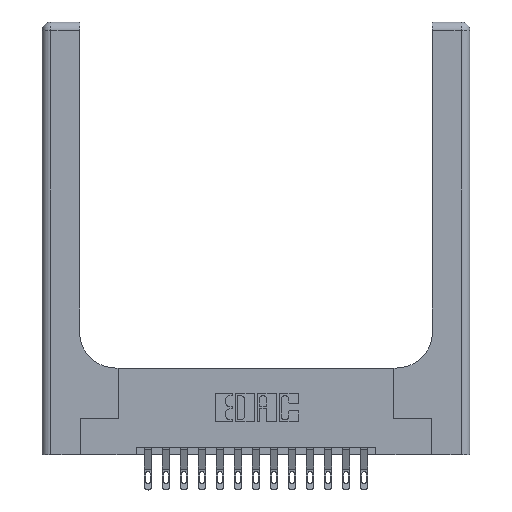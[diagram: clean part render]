
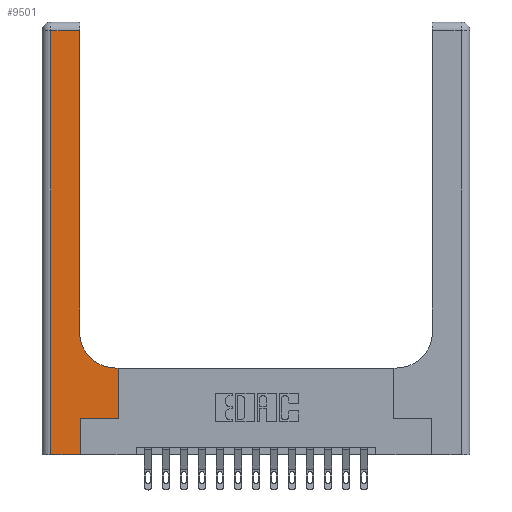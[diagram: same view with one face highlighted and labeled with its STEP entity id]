
A CAD part, top view. The second image highlights one B-rep face of the part: STEP entity #9501.
In plain terms, the highlighted planar face has unit normal (0, 0, 1).
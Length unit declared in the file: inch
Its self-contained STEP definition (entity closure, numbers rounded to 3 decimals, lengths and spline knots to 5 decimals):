
#253 = VECTOR ( 'NONE', #8707, 39.37008 ) ;
#255 = VERTEX_POINT ( 'NONE', #15334 ) ;
#496 = VERTEX_POINT ( 'NONE', #16063 ) ;
#743 = EDGE_CURVE ( 'NONE', #5864, #2166, #17079, .T. ) ;
#799 = CIRCLE ( 'NONE', #3580, 0.25 ) ;
#1097 = ORIENTED_EDGE ( 'NONE', *, *, #6140, .T. ) ;
#2155 = EDGE_CURVE ( 'NONE', #9867, #15164, #10991, .T. ) ;
#2166 = VERTEX_POINT ( 'NONE', #3751 ) ;
#2454 = DIRECTION ( 'NONE',  ( 1., 0., 0. ) ) ;
#2517 = CARTESIAN_POINT ( 'NONE',  ( 0.51, 0.85, 0.37 ) ) ;
#3580 = AXIS2_PLACEMENT_3D ( 'NONE', #2517, #16220, #2454 ) ;
#3751 = CARTESIAN_POINT ( 'NONE',  ( 0.06, 0., 0.37 ) ) ;
#4414 = ORIENTED_EDGE ( 'NONE', *, *, #14472, .T. ) ;
#4466 = ORIENTED_EDGE ( 'NONE', *, *, #5536, .T. ) ;
#4567 = CARTESIAN_POINT ( 'NONE',  ( 0.265, 0.25, 0.37 ) ) ;
#4694 = DIRECTION ( 'NONE',  ( 0., 1., 0. ) ) ;
#5116 = ORIENTED_EDGE ( 'NONE', *, *, #743, .T. ) ;
#5125 = VERTEX_POINT ( 'NONE', #13527 ) ;
#5138 = VECTOR ( 'NONE', #5755, 39.37008 ) ;
#5536 = EDGE_CURVE ( 'NONE', #2166, #9867, #12953, .T. ) ;
#5755 = DIRECTION ( 'NONE',  ( 0., 1., 0. ) ) ;
#5814 = CARTESIAN_POINT ( 'NONE',  ( 0.26, 2.94, 0.37 ) ) ;
#5864 = VERTEX_POINT ( 'NONE', #15288 ) ;
#5878 = CARTESIAN_POINT ( 'NONE',  ( 0.26, 3., 0.37 ) ) ;
#5992 = DIRECTION ( 'NONE',  ( -1., 0., 0. ) ) ;
#6130 = CARTESIAN_POINT ( 'NONE',  ( 0., 0., 0.37 ) ) ;
#6140 = EDGE_CURVE ( 'NONE', #15164, #6442, #11395, .T. ) ;
#6442 = VERTEX_POINT ( 'NONE', #11797 ) ;
#6445 = CARTESIAN_POINT ( 'NONE',  ( 0.265, 0.25, 0.37 ) ) ;
#6822 = LINE ( 'NONE', #11592, #13778 ) ;
#7314 = CARTESIAN_POINT ( 'NONE',  ( 0., 3., 0.37 ) ) ;
#7675 = VECTOR ( 'NONE', #10628, 39.37008 ) ;
#7740 = VERTEX_POINT ( 'NONE', #5814 ) ;
#8391 = PLANE ( 'NONE',  #9611 ) ;
#8683 = DIRECTION ( 'NONE',  ( 0., 0., -1. ) ) ;
#8707 = DIRECTION ( 'NONE',  ( -1., 0., 0. ) ) ;
#8830 = LINE ( 'NONE', #5878, #5138 ) ;
#9001 = VECTOR ( 'NONE', #10304, 39.37008 ) ;
#9010 = DIRECTION ( 'NONE',  ( 0., 1., 0. ) ) ;
#9082 = CARTESIAN_POINT ( 'NONE',  ( 0.265, 0., 0.37 ) ) ;
#9192 = EDGE_CURVE ( 'NONE', #7740, #5864, #13917, .T. ) ;
#9409 = ORIENTED_EDGE ( 'NONE', *, *, #10931, .T. ) ;
#9501 = ADVANCED_FACE ( 'NONE', ( #16927 ), #8391, .F. ) ;
#9611 = AXIS2_PLACEMENT_3D ( 'NONE', #7314, #8683, #5992 ) ;
#9620 = LINE ( 'NONE', #16177, #16108 ) ;
#9867 = VERTEX_POINT ( 'NONE', #12535 ) ;
#10184 = CARTESIAN_POINT ( 'NONE',  ( 0., 2.94, 0.37 ) ) ;
#10304 = DIRECTION ( 'NONE',  ( 1., 0., 0. ) ) ;
#10628 = DIRECTION ( 'NONE',  ( 1., 0., 0. ) ) ;
#10786 = ORIENTED_EDGE ( 'NONE', *, *, #17749, .T. ) ;
#10931 = EDGE_CURVE ( 'NONE', #255, #5125, #799, .T. ) ;
#10991 = LINE ( 'NONE', #9082, #17901 ) ;
#11395 = LINE ( 'NONE', #6445, #7675 ) ;
#11426 = EDGE_LOOP ( 'NONE', ( #4414, #17338, #5116, #4466, #15095, #1097, #14264, #10786, #9409 ) ) ;
#11592 = CARTESIAN_POINT ( 'NONE',  ( 0.26, 0.6, 0.37 ) ) ;
#11797 = CARTESIAN_POINT ( 'NONE',  ( 0.528, 0.25, 0.37 ) ) ;
#12535 = CARTESIAN_POINT ( 'NONE',  ( 0.265, 0., 0.37 ) ) ;
#12953 = LINE ( 'NONE', #6130, #9001 ) ;
#12960 = DIRECTION ( 'NONE',  ( 0., -1., 0. ) ) ;
#13216 = VECTOR ( 'NONE', #12960, 39.37008 ) ;
#13527 = CARTESIAN_POINT ( 'NONE',  ( 0.26, 0.85, 0.37 ) ) ;
#13778 = VECTOR ( 'NONE', #17260, 39.37008 ) ;
#13917 = LINE ( 'NONE', #10184, #253 ) ;
#14264 = ORIENTED_EDGE ( 'NONE', *, *, #17816, .T. ) ;
#14472 = EDGE_CURVE ( 'NONE', #5125, #7740, #8830, .T. ) ;
#15095 = ORIENTED_EDGE ( 'NONE', *, *, #2155, .T. ) ;
#15164 = VERTEX_POINT ( 'NONE', #4567 ) ;
#15288 = CARTESIAN_POINT ( 'NONE',  ( 0.06, 2.94, 0.37 ) ) ;
#15334 = CARTESIAN_POINT ( 'NONE',  ( 0.51, 0.6, 0.37 ) ) ;
#16063 = CARTESIAN_POINT ( 'NONE',  ( 0.528, 0.6, 0.37 ) ) ;
#16108 = VECTOR ( 'NONE', #9010, 39.37008 ) ;
#16177 = CARTESIAN_POINT ( 'NONE',  ( 0.528, 0.25, 0.37 ) ) ;
#16220 = DIRECTION ( 'NONE',  ( 0., 0., -1. ) ) ;
#16401 = CARTESIAN_POINT ( 'NONE',  ( 0.06, 3., 0.37 ) ) ;
#16927 = FACE_OUTER_BOUND ( 'NONE', #11426, .T. ) ;
#17079 = LINE ( 'NONE', #16401, #13216 ) ;
#17260 = DIRECTION ( 'NONE',  ( -1., 0., 0. ) ) ;
#17338 = ORIENTED_EDGE ( 'NONE', *, *, #9192, .T. ) ;
#17749 = EDGE_CURVE ( 'NONE', #496, #255, #6822, .T. ) ;
#17816 = EDGE_CURVE ( 'NONE', #6442, #496, #9620, .T. ) ;
#17901 = VECTOR ( 'NONE', #4694, 39.37008 ) ;
